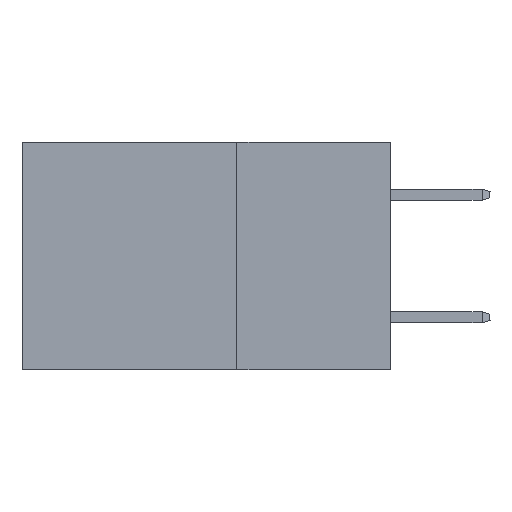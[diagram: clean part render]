
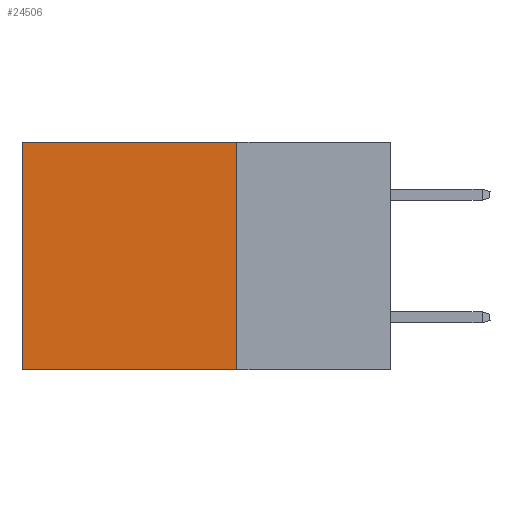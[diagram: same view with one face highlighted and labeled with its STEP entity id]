
A CAD part, left-side view. The second image highlights one B-rep face of the part: STEP entity #24506.
In plain terms, the highlighted planar face has unit normal (-1, 0, 0).
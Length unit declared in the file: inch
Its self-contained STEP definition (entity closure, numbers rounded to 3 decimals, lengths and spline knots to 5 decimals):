
#60 = CARTESIAN_POINT ( 'NONE',  ( 0.2875, 0.6, 0. ) ) ;
#317 = EDGE_LOOP ( 'NONE', ( #10735, #14478, #14332, #13018 ) ) ;
#1865 = VERTEX_POINT ( 'NONE', #28977 ) ;
#3310 = VERTEX_POINT ( 'NONE', #5714 ) ;
#3704 = DIRECTION ( 'NONE',  ( 0., 0., -1. ) ) ;
#5095 = AXIS2_PLACEMENT_3D ( 'NONE', #26527, #19110, #3704 ) ;
#5636 = CARTESIAN_POINT ( 'NONE',  ( 0.2875, 0.25, 0. ) ) ;
#5714 = CARTESIAN_POINT ( 'NONE',  ( 0.2875, 0.25, 0. ) ) ;
#10735 = ORIENTED_EDGE ( 'NONE', *, *, #28293, .T. ) ;
#11386 = PLANE ( 'NONE',  #5095 ) ;
#12283 = VECTOR ( 'NONE', #32897, 39.37008 ) ;
#13018 = ORIENTED_EDGE ( 'NONE', *, *, #29784, .T. ) ;
#13182 = VERTEX_POINT ( 'NONE', #28947 ) ;
#13390 = CARTESIAN_POINT ( 'NONE',  ( 0.2875, 0.25, 0. ) ) ;
#14119 = FACE_OUTER_BOUND ( 'NONE', #317, .T. ) ;
#14332 = ORIENTED_EDGE ( 'NONE', *, *, #17642, .F. ) ;
#14478 = ORIENTED_EDGE ( 'NONE', *, *, #25988, .F. ) ;
#15390 = CARTESIAN_POINT ( 'NONE',  ( 0.2875, 0.6, 0. ) ) ;
#15967 = DIRECTION ( 'NONE',  ( 0., 0., -1. ) ) ;
#16019 = LINE ( 'NONE', #17250, #27769 ) ;
#17250 = CARTESIAN_POINT ( 'NONE',  ( 0.2875, 0.25, -0.37 ) ) ;
#17642 = EDGE_CURVE ( 'NONE', #3310, #1865, #18670, .T. ) ;
#18670 = LINE ( 'NONE', #13390, #31921 ) ;
#19110 = DIRECTION ( 'NONE',  ( 1., 0., 0. ) ) ;
#22280 = DIRECTION ( 'NONE',  ( 0., 1., 0. ) ) ;
#24181 = VECTOR ( 'NONE', #30963, 39.37008 ) ;
#24506 = ADVANCED_FACE ( 'NONE', ( #14119 ), #11386, .F. ) ;
#25988 = EDGE_CURVE ( 'NONE', #1865, #13182, #16019, .T. ) ;
#26527 = CARTESIAN_POINT ( 'NONE',  ( 0.2875, 0.25, 0. ) ) ;
#27769 = VECTOR ( 'NONE', #22280, 39.37008 ) ;
#28293 = EDGE_CURVE ( 'NONE', #31685, #13182, #30783, .T. ) ;
#28947 = CARTESIAN_POINT ( 'NONE',  ( 0.2875, 0.6, -0.37 ) ) ;
#28977 = CARTESIAN_POINT ( 'NONE',  ( 0.2875, 0.25, -0.37 ) ) ;
#29784 = EDGE_CURVE ( 'NONE', #3310, #31685, #30812, .T. ) ;
#30783 = LINE ( 'NONE', #15390, #12283 ) ;
#30812 = LINE ( 'NONE', #5636, #24181 ) ;
#30963 = DIRECTION ( 'NONE',  ( 0., 1., 0. ) ) ;
#31685 = VERTEX_POINT ( 'NONE', #60 ) ;
#31921 = VECTOR ( 'NONE', #15967, 39.37008 ) ;
#32897 = DIRECTION ( 'NONE',  ( 0., 0., -1. ) ) ;
